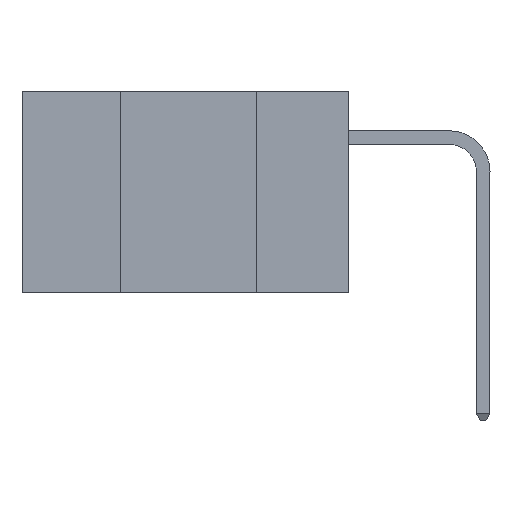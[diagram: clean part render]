
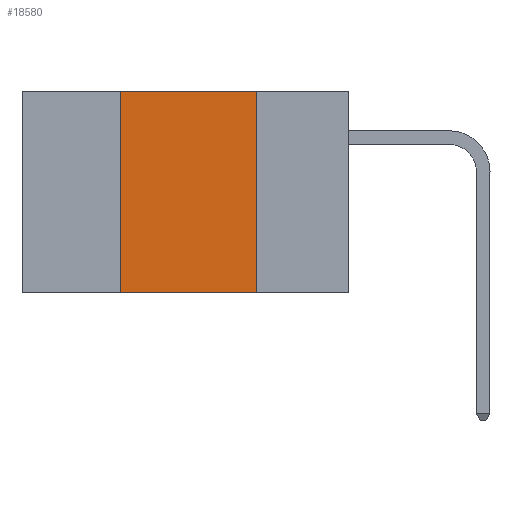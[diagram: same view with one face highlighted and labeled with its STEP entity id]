
A CAD part, left-side view. The second image highlights one B-rep face of the part: STEP entity #18580.
In plain terms, the highlighted planar face has unit normal (-1, 0, 0).
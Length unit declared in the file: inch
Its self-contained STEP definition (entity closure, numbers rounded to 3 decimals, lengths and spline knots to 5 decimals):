
#129 = CARTESIAN_POINT ( 'NONE',  ( 0., 0.42, 0. ) ) ;
#187 = DIRECTION ( 'NONE',  ( 0., -1., 0. ) ) ;
#327 = EDGE_CURVE ( 'NONE', #28964, #27412, #25428, .T. ) ;
#814 = EDGE_CURVE ( 'NONE', #24597, #27412, #9578, .T. ) ;
#1287 = VECTOR ( 'NONE', #187, 39.37008 ) ;
#2426 = DIRECTION ( 'NONE',  ( 0., 0., -1. ) ) ;
#5340 = ORIENTED_EDGE ( 'NONE', *, *, #5462, .F. ) ;
#5462 = EDGE_CURVE ( 'NONE', #32607, #28964, #15308, .T. ) ;
#6491 = ORIENTED_EDGE ( 'NONE', *, *, #814, .T. ) ;
#6667 = CARTESIAN_POINT ( 'NONE',  ( 0., 0.17, 0. ) ) ;
#7662 = VECTOR ( 'NONE', #23455, 39.37008 ) ;
#9578 = LINE ( 'NONE', #19837, #1287 ) ;
#9724 = LINE ( 'NONE', #34308, #30343 ) ;
#11438 = VECTOR ( 'NONE', #23374, 39.37008 ) ;
#13601 = FACE_OUTER_BOUND ( 'NONE', #33118, .T. ) ;
#13613 = ORIENTED_EDGE ( 'NONE', *, *, #35896, .F. ) ;
#15249 = CARTESIAN_POINT ( 'NONE',  ( 0., 0.6, 0. ) ) ;
#15308 = LINE ( 'NONE', #15249, #7662 ) ;
#16530 = PLANE ( 'NONE',  #29534 ) ;
#18580 = ADVANCED_FACE ( 'NONE', ( #13601 ), #16530, .F. ) ;
#19308 = DIRECTION ( 'NONE',  ( 1., 0., 0. ) ) ;
#19837 = CARTESIAN_POINT ( 'NONE',  ( 0., 0.6, -0.37 ) ) ;
#20607 = CARTESIAN_POINT ( 'NONE',  ( 0., 0.17, 0. ) ) ;
#23374 = DIRECTION ( 'NONE',  ( 0., 0., -1. ) ) ;
#23455 = DIRECTION ( 'NONE',  ( 0., -1., 0. ) ) ;
#24597 = VERTEX_POINT ( 'NONE', #25223 ) ;
#25223 = CARTESIAN_POINT ( 'NONE',  ( 0., 0.42, -0.37 ) ) ;
#25428 = LINE ( 'NONE', #20607, #11438 ) ;
#26825 = ORIENTED_EDGE ( 'NONE', *, *, #327, .F. ) ;
#27412 = VERTEX_POINT ( 'NONE', #33739 ) ;
#28861 = DIRECTION ( 'NONE',  ( 0., 0., 1. ) ) ;
#28964 = VERTEX_POINT ( 'NONE', #6667 ) ;
#29534 = AXIS2_PLACEMENT_3D ( 'NONE', #35787, #19308, #2426 ) ;
#30343 = VECTOR ( 'NONE', #28861, 39.37008 ) ;
#32607 = VERTEX_POINT ( 'NONE', #129 ) ;
#33118 = EDGE_LOOP ( 'NONE', ( #26825, #5340, #13613, #6491 ) ) ;
#33739 = CARTESIAN_POINT ( 'NONE',  ( 0., 0.17, -0.37 ) ) ;
#34308 = CARTESIAN_POINT ( 'NONE',  ( 0., 0.42, 0. ) ) ;
#35787 = CARTESIAN_POINT ( 'NONE',  ( 0., 0.6, 0. ) ) ;
#35896 = EDGE_CURVE ( 'NONE', #24597, #32607, #9724, .T. ) ;
